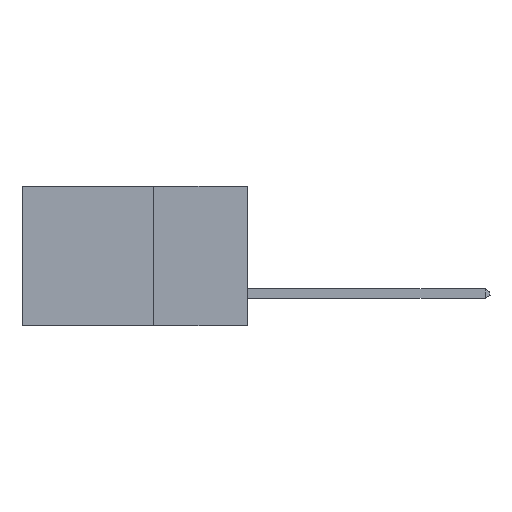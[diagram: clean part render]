
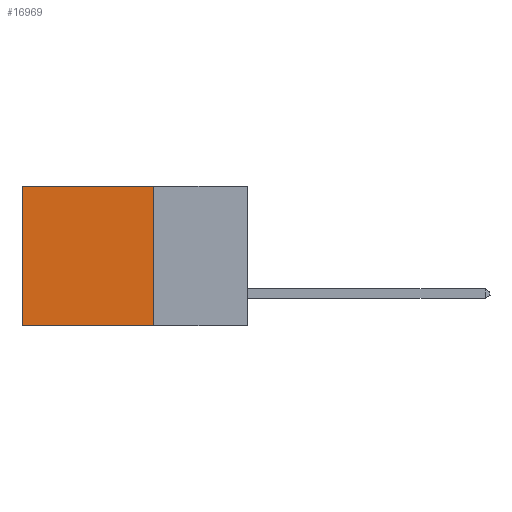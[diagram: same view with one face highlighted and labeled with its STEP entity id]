
A CAD part, left-side view. The second image highlights one B-rep face of the part: STEP entity #16969.
In plain terms, the highlighted planar face has unit normal (-1, 0, 0).
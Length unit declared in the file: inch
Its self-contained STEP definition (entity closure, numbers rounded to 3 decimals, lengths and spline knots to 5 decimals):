
#1437 = ORIENTED_EDGE ( 'NONE', *, *, #18596, .F. ) ;
#1568 = LINE ( 'NONE', #18941, #27207 ) ;
#1637 = VECTOR ( 'NONE', #27232, 39.37008 ) ;
#2953 = AXIS2_PLACEMENT_3D ( 'NONE', #23934, #11899, #18979 ) ;
#4227 = LINE ( 'NONE', #5506, #29523 ) ;
#4470 = CARTESIAN_POINT ( 'NONE',  ( 0.298, 0.25, 0. ) ) ;
#5506 = CARTESIAN_POINT ( 'NONE',  ( 0.298, 0.25, 0. ) ) ;
#5710 = VERTEX_POINT ( 'NONE', #6456 ) ;
#6456 = CARTESIAN_POINT ( 'NONE',  ( 0.298, 0.25, -0.37 ) ) ;
#7089 = CARTESIAN_POINT ( 'NONE',  ( 0.298, 0.6, 0. ) ) ;
#8835 = CARTESIAN_POINT ( 'NONE',  ( 0.298, 0.25, 0. ) ) ;
#10195 = LINE ( 'NONE', #8835, #12500 ) ;
#11504 = ORIENTED_EDGE ( 'NONE', *, *, #18087, .T. ) ;
#11899 = DIRECTION ( 'NONE',  ( 1., 0., 0. ) ) ;
#12209 = FACE_OUTER_BOUND ( 'NONE', #23524, .T. ) ;
#12500 = VECTOR ( 'NONE', #23341, 39.37008 ) ;
#15155 = ORIENTED_EDGE ( 'NONE', *, *, #30193, .F. ) ;
#16950 = PLANE ( 'NONE',  #2953 ) ;
#16969 = ADVANCED_FACE ( 'NONE', ( #12209 ), #16950, .F. ) ;
#18087 = EDGE_CURVE ( 'NONE', #21763, #19289, #4227, .T. ) ;
#18596 = EDGE_CURVE ( 'NONE', #21763, #5710, #10195, .T. ) ;
#18909 = CARTESIAN_POINT ( 'NONE',  ( 0.298, 0.25, -0.37 ) ) ;
#18941 = CARTESIAN_POINT ( 'NONE',  ( 0.298, 0.6, 0. ) ) ;
#18979 = DIRECTION ( 'NONE',  ( 0., 0., -1. ) ) ;
#19289 = VERTEX_POINT ( 'NONE', #7089 ) ;
#21763 = VERTEX_POINT ( 'NONE', #4470 ) ;
#23341 = DIRECTION ( 'NONE',  ( 0., 0., -1. ) ) ;
#23524 = EDGE_LOOP ( 'NONE', ( #28154, #15155, #1437, #11504 ) ) ;
#23914 = LINE ( 'NONE', #18909, #1637 ) ;
#23934 = CARTESIAN_POINT ( 'NONE',  ( 0.298, 0.25, 0. ) ) ;
#25535 = CARTESIAN_POINT ( 'NONE',  ( 0.298, 0.6, -0.37 ) ) ;
#27207 = VECTOR ( 'NONE', #30627, 39.37008 ) ;
#27232 = DIRECTION ( 'NONE',  ( 0., 1., 0. ) ) ;
#28123 = EDGE_CURVE ( 'NONE', #19289, #30903, #1568, .T. ) ;
#28154 = ORIENTED_EDGE ( 'NONE', *, *, #28123, .T. ) ;
#29493 = DIRECTION ( 'NONE',  ( 0., 1., 0. ) ) ;
#29523 = VECTOR ( 'NONE', #29493, 39.37008 ) ;
#30193 = EDGE_CURVE ( 'NONE', #5710, #30903, #23914, .T. ) ;
#30627 = DIRECTION ( 'NONE',  ( 0., 0., -1. ) ) ;
#30903 = VERTEX_POINT ( 'NONE', #25535 ) ;
